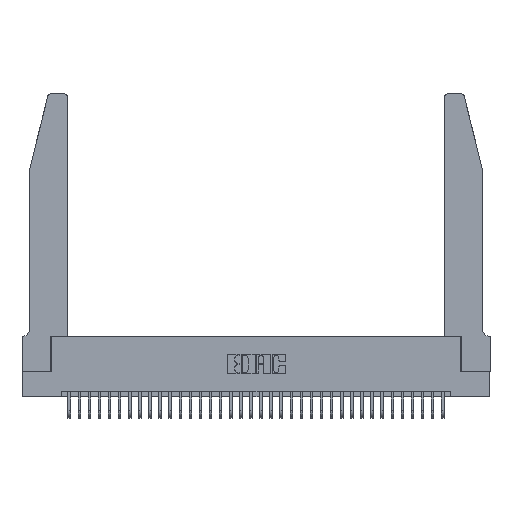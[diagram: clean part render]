
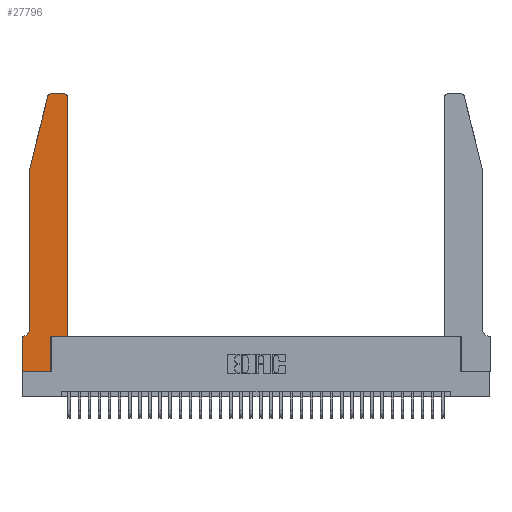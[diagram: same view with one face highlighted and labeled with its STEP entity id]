
A CAD part, top view. The second image highlights one B-rep face of the part: STEP entity #27796.
In plain terms, the highlighted planar face has unit normal (0, 0, 1).
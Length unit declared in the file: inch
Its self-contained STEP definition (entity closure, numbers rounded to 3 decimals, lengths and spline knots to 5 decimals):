
#628 = DIRECTION ( 'NONE',  ( -1., 0., 0. ) ) ;
#797 = EDGE_CURVE ( 'NONE', #32454, #24089, #31085, .T. ) ;
#889 = CARTESIAN_POINT ( 'NONE',  ( 0.0055, 0.42, 0.37 ) ) ;
#1435 = EDGE_CURVE ( 'NONE', #8144, #12329, #27951, .T. ) ;
#1436 = ORIENTED_EDGE ( 'NONE', *, *, #22704, .T. ) ;
#1518 = AXIS2_PLACEMENT_3D ( 'NONE', #11329, #11914, #23348 ) ;
#1739 = CIRCLE ( 'NONE', #5618, 0.03 ) ;
#2240 = CIRCLE ( 'NONE', #1518, 0.03 ) ;
#2399 = CARTESIAN_POINT ( 'NONE',  ( 0.4505, 0.35, 0.37 ) ) ;
#3096 = DIRECTION ( 'NONE',  ( 0., 1., 0. ) ) ;
#3423 = DIRECTION ( 'NONE',  ( -1., 0., 0. ) ) ;
#3651 = ORIENTED_EDGE ( 'NONE', *, *, #797, .T. ) ;
#3669 = VERTEX_POINT ( 'NONE', #21673 ) ;
#3844 = EDGE_CURVE ( 'NONE', #34138, #10669, #35307, .T. ) ;
#3954 = VERTEX_POINT ( 'NONE', #10627 ) ;
#4641 = ORIENTED_EDGE ( 'NONE', *, *, #29492, .T. ) ;
#5146 = ORIENTED_EDGE ( 'NONE', *, *, #3844, .T. ) ;
#5453 = ORIENTED_EDGE ( 'NONE', *, *, #15992, .T. ) ;
#5618 = AXIS2_PLACEMENT_3D ( 'NONE', #24743, #30450, #7865 ) ;
#5935 = ORIENTED_EDGE ( 'NONE', *, *, #24050, .T. ) ;
#6152 = CARTESIAN_POINT ( 'NONE',  ( 0.0755, 0.35, 0.37 ) ) ;
#6177 = EDGE_CURVE ( 'NONE', #36502, #9088, #25719, .T. ) ;
#6426 = CARTESIAN_POINT ( 'NONE',  ( 0., 0.35, 0.37 ) ) ;
#7250 = VECTOR ( 'NONE', #20051, 39.37008 ) ;
#7341 = DIRECTION ( 'NONE',  ( 0., 0., 1. ) ) ;
#7865 = DIRECTION ( 'NONE',  ( 1., 0., 0. ) ) ;
#8144 = VERTEX_POINT ( 'NONE', #18550 ) ;
#8319 = DIRECTION ( 'NONE',  ( 1., 0., 0. ) ) ;
#8428 = VECTOR ( 'NONE', #36351, 39.37008 ) ;
#8501 = CARTESIAN_POINT ( 'NONE',  ( 0., 0., 0.37 ) ) ;
#8866 = VECTOR ( 'NONE', #8319, 39.37008 ) ;
#9088 = VERTEX_POINT ( 'NONE', #13880 ) ;
#9818 = VECTOR ( 'NONE', #24876, 39.37008 ) ;
#10079 = AXIS2_PLACEMENT_3D ( 'NONE', #889, #23466, #628 ) ;
#10403 = FACE_OUTER_BOUND ( 'NONE', #11139, .T. ) ;
#10452 = CARTESIAN_POINT ( 'NONE',  ( 0., 0., 0.37 ) ) ;
#10601 = AXIS2_PLACEMENT_3D ( 'NONE', #35386, #7341, #35649 ) ;
#10627 = CARTESIAN_POINT ( 'NONE',  ( 0.4505, 2.72, 0.37 ) ) ;
#10669 = VERTEX_POINT ( 'NONE', #13802 ) ;
#10855 = CARTESIAN_POINT ( 'NONE',  ( 0.2605, 2.75, 0.37 ) ) ;
#11139 = EDGE_LOOP ( 'NONE', ( #5935, #12341, #1436, #5146, #19084, #30043, #35815, #27225, #4641, #3651, #5453, #15723 ) ) ;
#11329 = CARTESIAN_POINT ( 'NONE',  ( 0.284, 2.72, 0.37 ) ) ;
#11888 = VECTOR ( 'NONE', #3423, 39.37008 ) ;
#11914 = DIRECTION ( 'NONE',  ( 0., 0., 1. ) ) ;
#12329 = VERTEX_POINT ( 'NONE', #6426 ) ;
#12341 = ORIENTED_EDGE ( 'NONE', *, *, #12663, .T. ) ;
#12444 = LINE ( 'NONE', #10855, #8428 ) ;
#12663 = EDGE_CURVE ( 'NONE', #34269, #3669, #2240, .T. ) ;
#13618 = EDGE_CURVE ( 'NONE', #3954, #35935, #1739, .T. ) ;
#13787 = EDGE_CURVE ( 'NONE', #10669, #8144, #17616, .T. ) ;
#13802 = CARTESIAN_POINT ( 'NONE',  ( 0.0755, 0.42, 0.37 ) ) ;
#13880 = CARTESIAN_POINT ( 'NONE',  ( 0.2865, 0., 0.37 ) ) ;
#14408 = VECTOR ( 'NONE', #3096, 39.37008 ) ;
#15723 = ORIENTED_EDGE ( 'NONE', *, *, #13618, .T. ) ;
#15992 = EDGE_CURVE ( 'NONE', #24089, #3954, #26849, .T. ) ;
#16004 = VECTOR ( 'NONE', #21771, 39.37008 ) ;
#17188 = CARTESIAN_POINT ( 'NONE',  ( 0.4505, 0.35, 0.37 ) ) ;
#17325 = EDGE_CURVE ( 'NONE', #12329, #36502, #18679, .T. ) ;
#17616 = CIRCLE ( 'NONE', #10079, 0.07 ) ;
#18142 = VECTOR ( 'NONE', #28375, 39.37008 ) ;
#18336 = PLANE ( 'NONE',  #10601 ) ;
#18550 = CARTESIAN_POINT ( 'NONE',  ( 0.0055, 0.35, 0.37 ) ) ;
#18679 = LINE ( 'NONE', #10452, #16004 ) ;
#19084 = ORIENTED_EDGE ( 'NONE', *, *, #13787, .T. ) ;
#20051 = DIRECTION ( 'NONE',  ( -0.239, -0.971, 0. ) ) ;
#21673 = CARTESIAN_POINT ( 'NONE',  ( 0.25487, 2.72718, 0.37 ) ) ;
#21761 = CARTESIAN_POINT ( 'NONE',  ( 0.2865, 0.35, 0.37 ) ) ;
#21771 = DIRECTION ( 'NONE',  ( 0., -1., 0. ) ) ;
#22629 = CARTESIAN_POINT ( 'NONE',  ( 0.284, 2.75, 0.37 ) ) ;
#22704 = EDGE_CURVE ( 'NONE', #3669, #34138, #24103, .T. ) ;
#23348 = DIRECTION ( 'NONE',  ( 1., 0., 0. ) ) ;
#23466 = DIRECTION ( 'NONE',  ( 0., 0., -1. ) ) ;
#24050 = EDGE_CURVE ( 'NONE', #35935, #34269, #12444, .T. ) ;
#24089 = VERTEX_POINT ( 'NONE', #36599 ) ;
#24103 = LINE ( 'NONE', #28752, #7250 ) ;
#24743 = CARTESIAN_POINT ( 'NONE',  ( 0.4205, 2.72, 0.37 ) ) ;
#24876 = DIRECTION ( 'NONE',  ( 0., 1., 0. ) ) ;
#25122 = VECTOR ( 'NONE', #30809, 39.37008 ) ;
#25387 = CARTESIAN_POINT ( 'NONE',  ( 0.0755, 2., 0.37 ) ) ;
#25719 = LINE ( 'NONE', #8501, #18142 ) ;
#26191 = CARTESIAN_POINT ( 'NONE',  ( 0.2865, 0.35, 0.37 ) ) ;
#26786 = CARTESIAN_POINT ( 'NONE',  ( 0.4205, 2.75, 0.37 ) ) ;
#26849 = LINE ( 'NONE', #17188, #14408 ) ;
#27225 = ORIENTED_EDGE ( 'NONE', *, *, #6177, .T. ) ;
#27694 = CARTESIAN_POINT ( 'NONE',  ( 0.0755, 2., 0.37 ) ) ;
#27796 = ADVANCED_FACE ( 'NONE', ( #10403 ), #18336, .T. ) ;
#27951 = LINE ( 'NONE', #6152, #11888 ) ;
#28375 = DIRECTION ( 'NONE',  ( 1., 0., 0. ) ) ;
#28752 = CARTESIAN_POINT ( 'NONE',  ( 0.0755, 2., 0.37 ) ) ;
#29492 = EDGE_CURVE ( 'NONE', #9088, #32454, #32485, .T. ) ;
#30043 = ORIENTED_EDGE ( 'NONE', *, *, #1435, .T. ) ;
#30450 = DIRECTION ( 'NONE',  ( 0., 0., 1. ) ) ;
#30809 = DIRECTION ( 'NONE',  ( 0., -1., 0. ) ) ;
#31085 = LINE ( 'NONE', #2399, #8866 ) ;
#32454 = VERTEX_POINT ( 'NONE', #26191 ) ;
#32485 = LINE ( 'NONE', #21761, #9818 ) ;
#34138 = VERTEX_POINT ( 'NONE', #25387 ) ;
#34269 = VERTEX_POINT ( 'NONE', #22629 ) ;
#35193 = CARTESIAN_POINT ( 'NONE',  ( 0., 0., 0.37 ) ) ;
#35307 = LINE ( 'NONE', #27694, #25122 ) ;
#35386 = CARTESIAN_POINT ( 'NONE',  ( 0., 0.35, 0.37 ) ) ;
#35649 = DIRECTION ( 'NONE',  ( 1., 0., 0. ) ) ;
#35815 = ORIENTED_EDGE ( 'NONE', *, *, #17325, .T. ) ;
#35935 = VERTEX_POINT ( 'NONE', #26786 ) ;
#36351 = DIRECTION ( 'NONE',  ( -1., 0., 0. ) ) ;
#36502 = VERTEX_POINT ( 'NONE', #35193 ) ;
#36599 = CARTESIAN_POINT ( 'NONE',  ( 0.4505, 0.35, 0.37 ) ) ;
